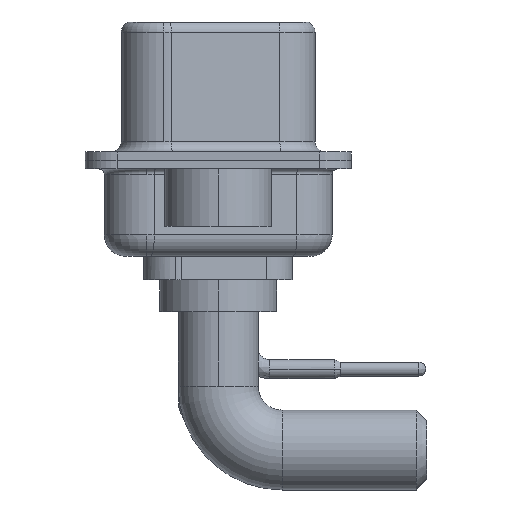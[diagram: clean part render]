
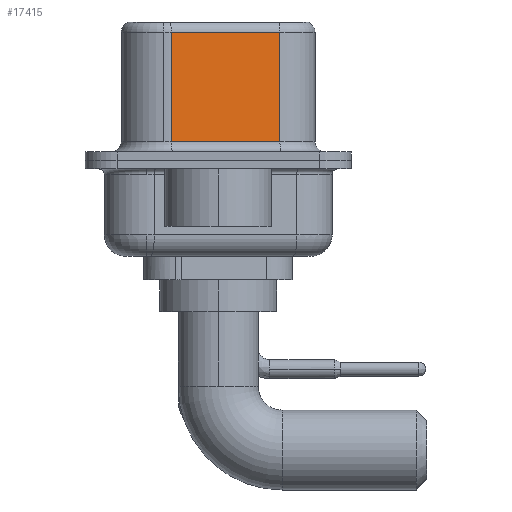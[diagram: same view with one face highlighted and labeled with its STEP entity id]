
A CAD part, left-side view. The second image highlights one B-rep face of the part: STEP entity #17415.
In plain terms, the highlighted planar face has unit normal (-0.985, -0.174, 0).
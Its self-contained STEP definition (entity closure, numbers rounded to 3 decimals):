
#801 = ORIENTED_EDGE ( 'NONE', *, *, #17908, .F. ) ;
#867 = PLANE ( 'NONE',  #8325 ) ;
#2509 = VECTOR ( 'NONE', #6959, 1000. ) ;
#2559 = CARTESIAN_POINT ( 'NONE',  ( 3.655, 2.203, 0.9 ) ) ;
#3560 = LINE ( 'NONE', #5555, #2509 ) ;
#4462 = CARTESIAN_POINT ( 'NONE',  ( 4.555, -2.897, 0.9 ) ) ;
#5555 = CARTESIAN_POINT ( 'NONE',  ( 4.555, -2.897, 6.02 ) ) ;
#6657 = EDGE_CURVE ( 'NONE', #8331, #18126, #3560, .T. ) ;
#6826 = EDGE_LOOP ( 'NONE', ( #801, #13459, #14112, #16288 ) ) ;
#6959 = DIRECTION ( 'NONE',  ( -0.174, 0.985, 0. ) ) ;
#7617 = VECTOR ( 'NONE', #7981, 1000. ) ;
#7849 = EDGE_CURVE ( 'NONE', #18126, #10877, #17403, .T. ) ;
#7981 = DIRECTION ( 'NONE',  ( 0.174, -0.985, 0. ) ) ;
#8325 = AXIS2_PLACEMENT_3D ( 'NONE', #9043, #10838, #15505 ) ;
#8331 = VERTEX_POINT ( 'NONE', #13104 ) ;
#9043 = CARTESIAN_POINT ( 'NONE',  ( 4.555, -2.897, 6.52 ) ) ;
#9452 = CARTESIAN_POINT ( 'NONE',  ( 3.655, 2.203, 6.52 ) ) ;
#10562 = VERTEX_POINT ( 'NONE', #14573 ) ;
#10838 = DIRECTION ( 'NONE',  ( 0.985, 0.174, 0. ) ) ;
#10877 = VERTEX_POINT ( 'NONE', #2559 ) ;
#12043 = VECTOR ( 'NONE', #19700, 1000. ) ;
#12538 = FACE_OUTER_BOUND ( 'NONE', #6826, .T. ) ;
#13104 = CARTESIAN_POINT ( 'NONE',  ( 4.555, -2.897, 6.02 ) ) ;
#13237 = LINE ( 'NONE', #16831, #12043 ) ;
#13459 = ORIENTED_EDGE ( 'NONE', *, *, #6657, .T. ) ;
#14112 = ORIENTED_EDGE ( 'NONE', *, *, #7849, .T. ) ;
#14127 = DIRECTION ( 'NONE',  ( 0., 0., -1. ) ) ;
#14573 = CARTESIAN_POINT ( 'NONE',  ( 4.555, -2.897, 0.9 ) ) ;
#15123 = EDGE_CURVE ( 'NONE', #10877, #10562, #19213, .T. ) ;
#15505 = DIRECTION ( 'NONE',  ( -0.174, 0.985, 0. ) ) ;
#16288 = ORIENTED_EDGE ( 'NONE', *, *, #15123, .T. ) ;
#16831 = CARTESIAN_POINT ( 'NONE',  ( 4.555, -2.897, 6.52 ) ) ;
#17403 = LINE ( 'NONE', #9452, #18776 ) ;
#17415 = ADVANCED_FACE ( 'NONE', ( #12538 ), #867, .F. ) ;
#17908 = EDGE_CURVE ( 'NONE', #8331, #10562, #13237, .T. ) ;
#18126 = VERTEX_POINT ( 'NONE', #20756 ) ;
#18776 = VECTOR ( 'NONE', #14127, 1000. ) ;
#19213 = LINE ( 'NONE', #4462, #7617 ) ;
#19700 = DIRECTION ( 'NONE',  ( 0., 0., -1. ) ) ;
#20756 = CARTESIAN_POINT ( 'NONE',  ( 3.655, 2.203, 6.02 ) ) ;
